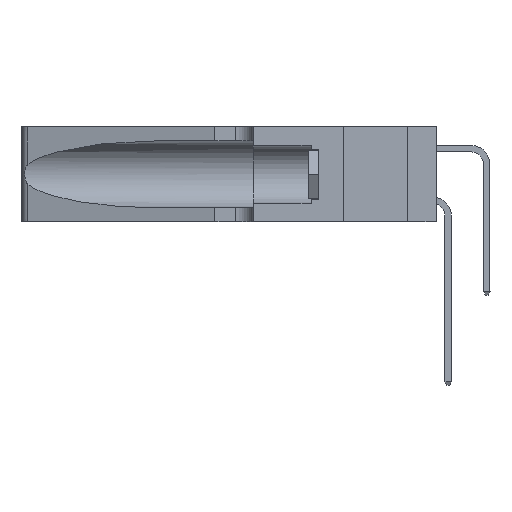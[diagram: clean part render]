
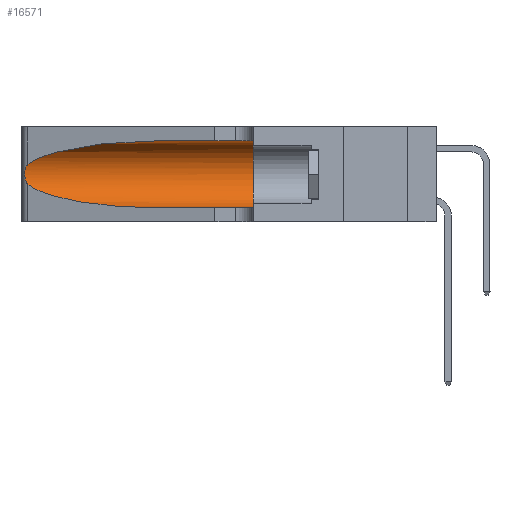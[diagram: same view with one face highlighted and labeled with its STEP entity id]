
A CAD part, left-side view. The second image highlights one B-rep face of the part: STEP entity #16571.
In plain terms, the highlighted cylindrical face has radius 3.308 mm (diameter 6.617 mm), a partial arc.
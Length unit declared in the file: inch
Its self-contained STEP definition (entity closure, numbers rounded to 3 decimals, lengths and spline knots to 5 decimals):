
#549 = CARTESIAN_POINT ( 'NONE',  ( 0.25487, 1.22718, 0.14631 ) ) ;
#767 = CARTESIAN_POINT ( 'NONE',  ( 0.25487, 1.22718, 0.22369 ) ) ;
#792 = CARTESIAN_POINT ( 'NONE',  ( 0.2373, 1.15595, 0.28018 ) ) ;
#880 = CARTESIAN_POINT ( 'NONE',  ( 0.25856, 1.23593, 0.16098 ) ) ;
#1993 = DIRECTION ( 'NONE',  ( 0., 1., 0. ) ) ;
#2032 = ORIENTED_EDGE ( 'NONE', *, *, #7011, .T. ) ;
#2047 = CARTESIAN_POINT ( 'NONE',  ( 0.25487, 1.22718, 0.14631 ) ) ;
#3191 = CYLINDRICAL_SURFACE ( 'NONE', #27512, 0.13025 ) ;
#3327 = EDGE_CURVE ( 'NONE', #5446, #14609, #5768, .T. ) ;
#3571 = CARTESIAN_POINT ( 'NONE',  ( 0.25487, 1.22718, 0.22369 ) ) ;
#3714 = CARTESIAN_POINT ( 'NONE',  ( 0.1305, 0.72297, 0.05475 ) ) ;
#3904 = CARTESIAN_POINT ( 'NONE',  ( 0.18966, 0.96281, 0.31525 ) ) ;
#4924 = AXIS2_PLACEMENT_3D ( 'NONE', #13163, #1993, #18591 ) ;
#5446 = VERTEX_POINT ( 'NONE', #34922 ) ;
#5768 = CIRCLE ( 'NONE', #4924, 0.13025 ) ;
#5912 = CARTESIAN_POINT ( 'NONE',  ( 0.25487, 1.22718, 0.14631 ) ) ;
#6867 = VERTEX_POINT ( 'NONE', #25718 ) ;
#7011 = EDGE_CURVE ( 'NONE', #6867, #14609, #21552, .T. ) ;
#8291 =( BOUNDED_CURVE ( )  B_SPLINE_CURVE ( 3, ( #33768, #3904, #792, #3571 ),
 .UNSPECIFIED., .F., .F. ) 
 B_SPLINE_CURVE_WITH_KNOTS ( ( 4, 4 ),
 ( 1.5708, 2.84003 ),
 .UNSPECIFIED. ) 
 CURVE ( )  GEOMETRIC_REPRESENTATION_ITEM ( )  RATIONAL_B_SPLINE_CURVE ( ( 1., 0.87, 0.87, 1. ) ) 
 REPRESENTATION_ITEM ( '' )  );
#8333 = ORIENTED_EDGE ( 'NONE', *, *, #3327, .F. ) ;
#8648 = VERTEX_POINT ( 'NONE', #21054 ) ;
#9073 = EDGE_LOOP ( 'NONE', ( #30763, #18054, #32462, #2032, #8333, #21643 ) ) ;
#9085 = CARTESIAN_POINT ( 'NONE',  ( 0.26075, 1.23896, 0.178 ) ) ;
#9137 = CARTESIAN_POINT ( 'NONE',  ( 0.18966, 0.96281, 0.05475 ) ) ;
#11803 = CARTESIAN_POINT ( 'NONE',  ( 0.25639, 1.23186, 0.15144 ) ) ;
#11916 = CARTESIAN_POINT ( 'NONE',  ( 0.25787, 1.23484, 0.2124 ) ) ;
#12113 = CARTESIAN_POINT ( 'NONE',  ( 0.25487, 1.22718, 0.22369 ) ) ;
#12176 = FACE_OUTER_BOUND ( 'NONE', #9073, .T. ) ;
#12868 = EDGE_CURVE ( 'NONE', #8648, #19631, #8291, .T. ) ;
#13163 = CARTESIAN_POINT ( 'NONE',  ( 0.1305, 0.35, 0.185 ) ) ;
#13249 = VERTEX_POINT ( 'NONE', #2047 ) ;
#14134 = EDGE_CURVE ( 'NONE', #13249, #6867, #18416, .T. ) ;
#14609 = VERTEX_POINT ( 'NONE', #22834 ) ;
#16571 = ADVANCED_FACE ( 'NONE', ( #12176 ), #3191, .F. ) ;
#17100 = EDGE_CURVE ( 'NONE', #19631, #13249, #34991, .T. ) ;
#17767 = DIRECTION ( 'NONE',  ( 0., -1., 0. ) ) ;
#17770 = DIRECTION ( 'NONE',  ( 0., -1., 0. ) ) ;
#18054 = ORIENTED_EDGE ( 'NONE', *, *, #17100, .T. ) ;
#18416 =( BOUNDED_CURVE ( )  B_SPLINE_CURVE ( 3, ( #5912, #18771, #9137, #3714 ),
 .UNSPECIFIED., .F., .F. ) 
 B_SPLINE_CURVE_WITH_KNOTS ( ( 4, 4 ),
 ( 3.44316, 4.71239 ),
 .UNSPECIFIED. ) 
 CURVE ( )  GEOMETRIC_REPRESENTATION_ITEM ( )  RATIONAL_B_SPLINE_CURVE ( ( 1., 0.87, 0.87, 1. ) ) 
 REPRESENTATION_ITEM ( '' )  );
#18591 = DIRECTION ( 'NONE',  ( 0., 0., 1. ) ) ;
#18771 = CARTESIAN_POINT ( 'NONE',  ( 0.2373, 1.15595, 0.08982 ) ) ;
#19414 = VECTOR ( 'NONE', #17770, 39.37008 ) ;
#19631 = VERTEX_POINT ( 'NONE', #12113 ) ;
#20294 = VECTOR ( 'NONE', #17767, 39.37008 ) ;
#21054 = CARTESIAN_POINT ( 'NONE',  ( 0.1305, 0.72297, 0.31525 ) ) ;
#21552 = LINE ( 'NONE', #34253, #19414 ) ;
#21643 = ORIENTED_EDGE ( 'NONE', *, *, #22870, .F. ) ;
#22580 = CARTESIAN_POINT ( 'NONE',  ( 0.25854, 1.2359, 0.20912 ) ) ;
#22687 = CARTESIAN_POINT ( 'NONE',  ( 0.25555, 1.22994, 0.2215 ) ) ;
#22804 = CARTESIAN_POINT ( 'NONE',  ( 0.26017, 1.23833, 0.17102 ) ) ;
#22834 = CARTESIAN_POINT ( 'NONE',  ( 0.1305, 0.35, 0.05475 ) ) ;
#22870 = EDGE_CURVE ( 'NONE', #8648, #5446, #28912, .T. ) ;
#22877 = CARTESIAN_POINT ( 'NONE',  ( 0.1305, 1.61858, 0.185 ) ) ;
#25445 = CARTESIAN_POINT ( 'NONE',  ( 0.25789, 1.23486, 0.15765 ) ) ;
#25718 = CARTESIAN_POINT ( 'NONE',  ( 0.1305, 0.72297, 0.05475 ) ) ;
#27512 = AXIS2_PLACEMENT_3D ( 'NONE', #22877, #33927, #30925 ) ;
#28113 = CARTESIAN_POINT ( 'NONE',  ( 0.26018, 1.23835, 0.19895 ) ) ;
#28912 = LINE ( 'NONE', #34248, #20294 ) ;
#30763 = ORIENTED_EDGE ( 'NONE', *, *, #12868, .T. ) ;
#30925 = DIRECTION ( 'NONE',  ( 0., 0., -1. ) ) ;
#31088 = CARTESIAN_POINT ( 'NONE',  ( 0.25555, 1.22993, 0.14849 ) ) ;
#31212 = CARTESIAN_POINT ( 'NONE',  ( 0.26075, 1.23896, 0.19203 ) ) ;
#32462 = ORIENTED_EDGE ( 'NONE', *, *, #14134, .T. ) ;
#33768 = CARTESIAN_POINT ( 'NONE',  ( 0.1305, 0.72297, 0.31525 ) ) ;
#33867 = CARTESIAN_POINT ( 'NONE',  ( 0.25639, 1.23184, 0.21858 ) ) ;
#33927 = DIRECTION ( 'NONE',  ( 0., -1., 0. ) ) ;
#34248 = CARTESIAN_POINT ( 'NONE',  ( 0.1305, 1.61858, 0.31525 ) ) ;
#34253 = CARTESIAN_POINT ( 'NONE',  ( 0.1305, 1.61858, 0.05475 ) ) ;
#34922 = CARTESIAN_POINT ( 'NONE',  ( 0.1305, 0.35, 0.31525 ) ) ;
#34991 = B_SPLINE_CURVE_WITH_KNOTS ( 'NONE', 3,
 ( #767, #22687, #33867, #11916, #22580, #28113, #31212, #9085, #22804, #880, #25445, #11803, #31088, #549 ),
 .UNSPECIFIED., .F., .F.,
 ( 4, 2, 2, 2, 2, 2, 4 ),
 ( 0., 0.00027, 0.00053, 0.00107, 0.0016, 0.00187, 0.00214 ),
 .UNSPECIFIED. ) ;
